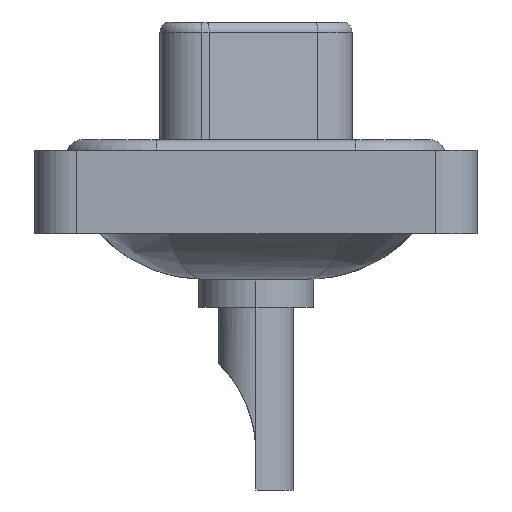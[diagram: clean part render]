
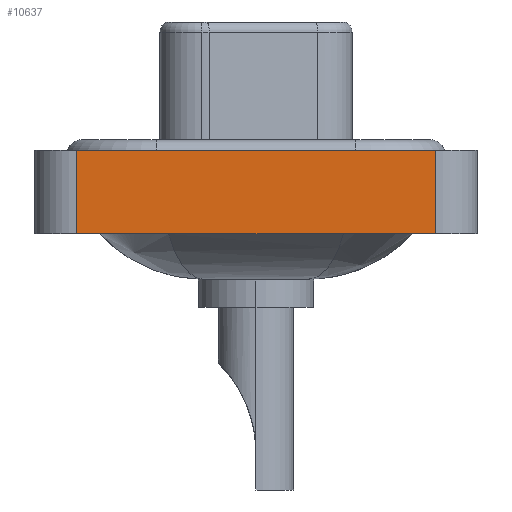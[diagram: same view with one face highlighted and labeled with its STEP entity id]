
A CAD part, left-side view. The second image highlights one B-rep face of the part: STEP entity #10637.
In plain terms, the highlighted planar face has unit normal (-1, 0, 0).
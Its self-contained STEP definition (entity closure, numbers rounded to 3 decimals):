
#567 = DIRECTION ( 'NONE',  ( 0., 0., 1. ) ) ;
#627 = CARTESIAN_POINT ( 'NONE',  ( -7.3, -8.55, -3.6 ) ) ;
#1036 = VERTEX_POINT ( 'NONE', #627 ) ;
#1671 = VERTEX_POINT ( 'NONE', #4920 ) ;
#1931 = DIRECTION ( 'NONE',  ( -1., 0., 0. ) ) ;
#2099 = LINE ( 'NONE', #8814, #2586 ) ;
#2586 = VECTOR ( 'NONE', #15362, 1000. ) ;
#2930 = CARTESIAN_POINT ( 'NONE',  ( -7.3, 8.55, 0.4 ) ) ;
#3041 = CARTESIAN_POINT ( 'NONE',  ( -7.3, -8.55, -3.6 ) ) ;
#3171 = ORIENTED_EDGE ( 'NONE', *, *, #16391, .F. ) ;
#3996 = DIRECTION ( 'NONE',  ( 0., 0., 1. ) ) ;
#4764 = VECTOR ( 'NONE', #3996, 1000. ) ;
#4920 = CARTESIAN_POINT ( 'NONE',  ( -7.3, 8.55, -3.6 ) ) ;
#5643 = ORIENTED_EDGE ( 'NONE', *, *, #12313, .T. ) ;
#5968 = FACE_OUTER_BOUND ( 'NONE', #12744, .T. ) ;
#7503 = LINE ( 'NONE', #8872, #9179 ) ;
#8227 = LINE ( 'NONE', #15901, #11384 ) ;
#8314 = DIRECTION ( 'NONE',  ( 0., -1., 0. ) ) ;
#8814 = CARTESIAN_POINT ( 'NONE',  ( -7.3, 8.55, -3.6 ) ) ;
#8872 = CARTESIAN_POINT ( 'NONE',  ( -7.3, -8.55, -3.6 ) ) ;
#9179 = VECTOR ( 'NONE', #14066, 1000. ) ;
#9582 = EDGE_CURVE ( 'NONE', #1671, #16003, #2099, .T. ) ;
#10637 = ADVANCED_FACE ( 'NONE', ( #5968 ), #11211, .T. ) ;
#10783 = ORIENTED_EDGE ( 'NONE', *, *, #9582, .F. ) ;
#11211 = PLANE ( 'NONE',  #13591 ) ;
#11384 = VECTOR ( 'NONE', #8314, 1000. ) ;
#12313 = EDGE_CURVE ( 'NONE', #1671, #1036, #7503, .T. ) ;
#12744 = EDGE_LOOP ( 'NONE', ( #15870, #3171, #10783, #5643 ) ) ;
#12829 = LINE ( 'NONE', #16932, #4764 ) ;
#13591 = AXIS2_PLACEMENT_3D ( 'NONE', #3041, #1931, #567 ) ;
#14066 = DIRECTION ( 'NONE',  ( 0., -1., 0. ) ) ;
#14959 = EDGE_CURVE ( 'NONE', #1036, #15128, #12829, .T. ) ;
#15128 = VERTEX_POINT ( 'NONE', #16406 ) ;
#15362 = DIRECTION ( 'NONE',  ( 0., 0., 1. ) ) ;
#15870 = ORIENTED_EDGE ( 'NONE', *, *, #14959, .T. ) ;
#15901 = CARTESIAN_POINT ( 'NONE',  ( -7.3, -8.55, 0.4 ) ) ;
#16003 = VERTEX_POINT ( 'NONE', #2930 ) ;
#16391 = EDGE_CURVE ( 'NONE', #16003, #15128, #8227, .T. ) ;
#16406 = CARTESIAN_POINT ( 'NONE',  ( -7.3, -8.55, 0.4 ) ) ;
#16932 = CARTESIAN_POINT ( 'NONE',  ( -7.3, -8.55, -3.6 ) ) ;
